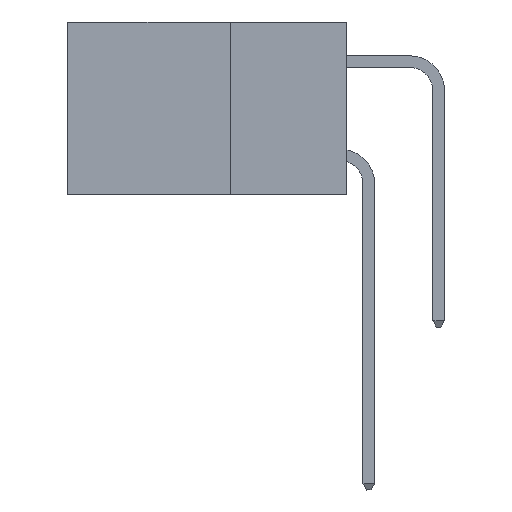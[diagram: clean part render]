
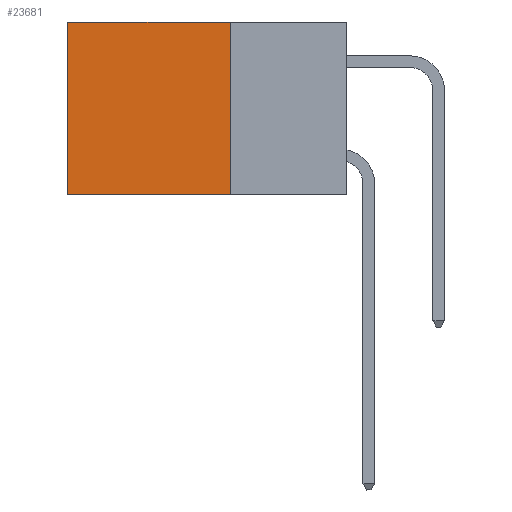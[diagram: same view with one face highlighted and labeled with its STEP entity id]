
A CAD part, left-side view. The second image highlights one B-rep face of the part: STEP entity #23681.
In plain terms, the highlighted planar face has unit normal (-1, 0, 0).
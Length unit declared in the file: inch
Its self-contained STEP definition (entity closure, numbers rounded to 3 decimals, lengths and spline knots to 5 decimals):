
#2321 = EDGE_CURVE ( 'NONE', #34352, #10356, #27971, .T. ) ;
#3668 = VECTOR ( 'NONE', #18805, 39.37008 ) ;
#4189 = VERTEX_POINT ( 'NONE', #19396 ) ;
#5252 = DIRECTION ( 'NONE',  ( 0., 1., 0. ) ) ;
#6574 = VECTOR ( 'NONE', #29966, 39.37008 ) ;
#7596 = CARTESIAN_POINT ( 'NONE',  ( 0.2875, 0.25, 0. ) ) ;
#8735 = CARTESIAN_POINT ( 'NONE',  ( 0.2875, 0.25, 0. ) ) ;
#9852 = LINE ( 'NONE', #21189, #16965 ) ;
#9984 = CARTESIAN_POINT ( 'NONE',  ( 0.2875, 0.25, -0.37 ) ) ;
#10275 = DIRECTION ( 'NONE',  ( 1., 0., 0. ) ) ;
#10356 = VERTEX_POINT ( 'NONE', #9984 ) ;
#13992 = ORIENTED_EDGE ( 'NONE', *, *, #2321, .F. ) ;
#16140 = CARTESIAN_POINT ( 'NONE',  ( 0.2875, 0.25, -0.37 ) ) ;
#16711 = CARTESIAN_POINT ( 'NONE',  ( 0.2875, 0.6, 0. ) ) ;
#16965 = VECTOR ( 'NONE', #5252, 39.37008 ) ;
#17129 = ORIENTED_EDGE ( 'NONE', *, *, #17433, .T. ) ;
#17433 = EDGE_CURVE ( 'NONE', #31029, #4189, #34049, .T. ) ;
#18771 = CARTESIAN_POINT ( 'NONE',  ( 0.2875, 0.25, 0. ) ) ;
#18805 = DIRECTION ( 'NONE',  ( 0., 1., 0. ) ) ;
#19396 = CARTESIAN_POINT ( 'NONE',  ( 0.2875, 0.6, -0.37 ) ) ;
#19633 = ORIENTED_EDGE ( 'NONE', *, *, #24461, .T. ) ;
#19866 = ORIENTED_EDGE ( 'NONE', *, *, #27155, .F. ) ;
#21189 = CARTESIAN_POINT ( 'NONE',  ( 0.2875, 0.25, 0. ) ) ;
#21331 = CARTESIAN_POINT ( 'NONE',  ( 0.2875, 0.6, 0. ) ) ;
#23681 = ADVANCED_FACE ( 'NONE', ( #29033 ), #26243, .F. ) ;
#24461 = EDGE_CURVE ( 'NONE', #34352, #31029, #9852, .T. ) ;
#25237 = AXIS2_PLACEMENT_3D ( 'NONE', #7596, #10275, #28921 ) ;
#26243 = PLANE ( 'NONE',  #25237 ) ;
#26290 = VECTOR ( 'NONE', #30400, 39.37008 ) ;
#27155 = EDGE_CURVE ( 'NONE', #10356, #4189, #31995, .T. ) ;
#27626 = EDGE_LOOP ( 'NONE', ( #17129, #19866, #13992, #19633 ) ) ;
#27971 = LINE ( 'NONE', #8735, #26290 ) ;
#28921 = DIRECTION ( 'NONE',  ( 0., 0., -1. ) ) ;
#29033 = FACE_OUTER_BOUND ( 'NONE', #27626, .T. ) ;
#29966 = DIRECTION ( 'NONE',  ( 0., 0., -1. ) ) ;
#30400 = DIRECTION ( 'NONE',  ( 0., 0., -1. ) ) ;
#31029 = VERTEX_POINT ( 'NONE', #21331 ) ;
#31995 = LINE ( 'NONE', #16140, #3668 ) ;
#34049 = LINE ( 'NONE', #16711, #6574 ) ;
#34352 = VERTEX_POINT ( 'NONE', #18771 ) ;
